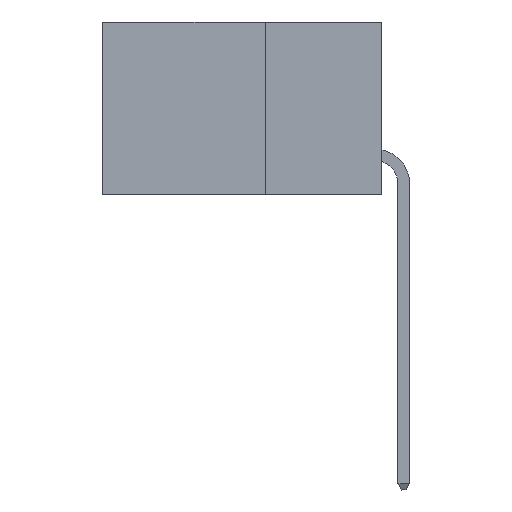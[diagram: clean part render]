
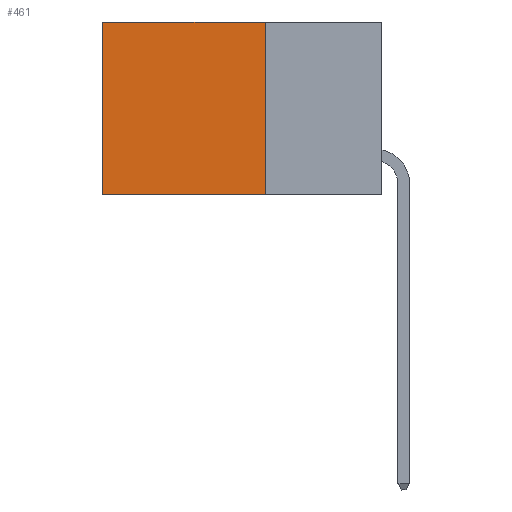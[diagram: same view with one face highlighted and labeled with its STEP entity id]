
A CAD part, left-side view. The second image highlights one B-rep face of the part: STEP entity #461.
In plain terms, the highlighted planar face has unit normal (-1, 0, 0).
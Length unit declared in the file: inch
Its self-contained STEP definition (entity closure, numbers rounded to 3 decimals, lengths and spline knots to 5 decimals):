
#98 = EDGE_CURVE ( 'NONE', #7464, #3144, #4611, .T. ) ;
#326 = EDGE_CURVE ( 'NONE', #11537, #7871, #723, .T. ) ;
#461 = ADVANCED_FACE ( 'NONE', ( #2302 ), #5323, .F. ) ;
#723 = LINE ( 'NONE', #8538, #8173 ) ;
#974 = CARTESIAN_POINT ( 'NONE',  ( 0.2875, 0.25, 0. ) ) ;
#2109 = CARTESIAN_POINT ( 'NONE',  ( 0.2875, 0.25, -0.37 ) ) ;
#2129 = ORIENTED_EDGE ( 'NONE', *, *, #98, .F. ) ;
#2302 = FACE_OUTER_BOUND ( 'NONE', #5465, .T. ) ;
#2321 = AXIS2_PLACEMENT_3D ( 'NONE', #11842, #6282, #4500 ) ;
#3144 = VERTEX_POINT ( 'NONE', #3474 ) ;
#3378 = VECTOR ( 'NONE', #7211, 39.37008 ) ;
#3474 = CARTESIAN_POINT ( 'NONE',  ( 0.2875, 0.6, -0.37 ) ) ;
#3479 = ORIENTED_EDGE ( 'NONE', *, *, #9171, .T. ) ;
#3607 = CARTESIAN_POINT ( 'NONE',  ( 0.2875, 0.6, 0. ) ) ;
#4041 = VECTOR ( 'NONE', #6551, 39.37008 ) ;
#4500 = DIRECTION ( 'NONE',  ( 0., 0., -1. ) ) ;
#4521 = DIRECTION ( 'NONE',  ( 0., 0., -1. ) ) ;
#4611 = LINE ( 'NONE', #2109, #4041 ) ;
#4665 = LINE ( 'NONE', #3607, #3378 ) ;
#4689 = CARTESIAN_POINT ( 'NONE',  ( 0.2875, 0.6, 0. ) ) ;
#5180 = LINE ( 'NONE', #974, #8751 ) ;
#5323 = PLANE ( 'NONE',  #2321 ) ;
#5465 = EDGE_LOOP ( 'NONE', ( #3479, #2129, #6213, #9993 ) ) ;
#6213 = ORIENTED_EDGE ( 'NONE', *, *, #11312, .F. ) ;
#6282 = DIRECTION ( 'NONE',  ( 1., 0., 0. ) ) ;
#6551 = DIRECTION ( 'NONE',  ( 0., 1., 0. ) ) ;
#7211 = DIRECTION ( 'NONE',  ( 0., 0., -1. ) ) ;
#7464 = VERTEX_POINT ( 'NONE', #8277 ) ;
#7871 = VERTEX_POINT ( 'NONE', #4689 ) ;
#8173 = VECTOR ( 'NONE', #11379, 39.37008 ) ;
#8277 = CARTESIAN_POINT ( 'NONE',  ( 0.2875, 0.25, -0.37 ) ) ;
#8538 = CARTESIAN_POINT ( 'NONE',  ( 0.2875, 0.25, 0. ) ) ;
#8751 = VECTOR ( 'NONE', #4521, 39.37008 ) ;
#9171 = EDGE_CURVE ( 'NONE', #7871, #3144, #4665, .T. ) ;
#9993 = ORIENTED_EDGE ( 'NONE', *, *, #326, .T. ) ;
#11312 = EDGE_CURVE ( 'NONE', #11537, #7464, #5180, .T. ) ;
#11379 = DIRECTION ( 'NONE',  ( 0., 1., 0. ) ) ;
#11500 = CARTESIAN_POINT ( 'NONE',  ( 0.2875, 0.25, 0. ) ) ;
#11537 = VERTEX_POINT ( 'NONE', #11500 ) ;
#11842 = CARTESIAN_POINT ( 'NONE',  ( 0.2875, 0.25, 0. ) ) ;
